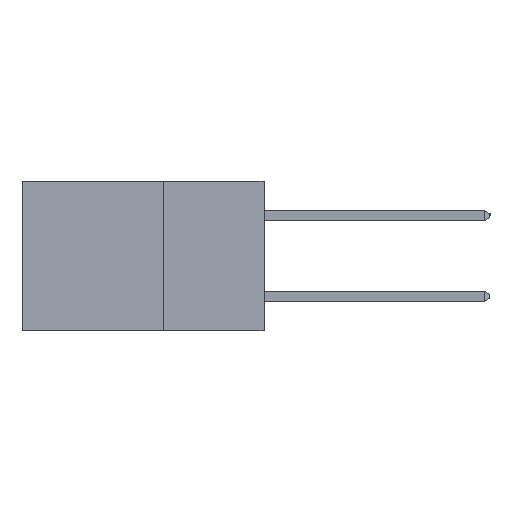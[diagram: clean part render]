
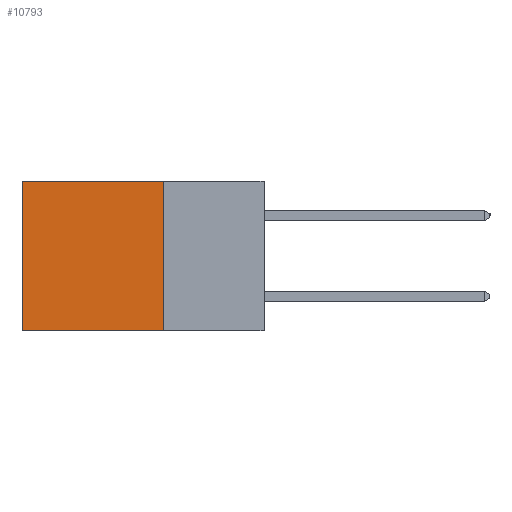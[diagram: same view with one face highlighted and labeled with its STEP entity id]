
A CAD part, left-side view. The second image highlights one B-rep face of the part: STEP entity #10793.
In plain terms, the highlighted planar face has unit normal (-1, 0, 0).
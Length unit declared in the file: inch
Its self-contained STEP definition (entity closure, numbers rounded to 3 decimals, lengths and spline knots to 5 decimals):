
#850 = VERTEX_POINT ( 'NONE', #3762 ) ;
#2221 = VECTOR ( 'NONE', #15880, 39.37008 ) ;
#2418 = CARTESIAN_POINT ( 'NONE',  ( 0.2615, 0.25, -0.37 ) ) ;
#2603 = ORIENTED_EDGE ( 'NONE', *, *, #13278, .T. ) ;
#2733 = ORIENTED_EDGE ( 'NONE', *, *, #13784, .T. ) ;
#2895 = VERTEX_POINT ( 'NONE', #5074 ) ;
#3762 = CARTESIAN_POINT ( 'NONE',  ( 0.2615, 0.25, 0. ) ) ;
#4779 = VERTEX_POINT ( 'NONE', #9271 ) ;
#4970 = CARTESIAN_POINT ( 'NONE',  ( 0.2615, 0.25, -0.37 ) ) ;
#5074 = CARTESIAN_POINT ( 'NONE',  ( 0.2615, 0.25, -0.37 ) ) ;
#6225 = LINE ( 'NONE', #11786, #14156 ) ;
#7426 = AXIS2_PLACEMENT_3D ( 'NONE', #8160, #14852, #13680 ) ;
#7540 = EDGE_CURVE ( 'NONE', #850, #2895, #10992, .T. ) ;
#8160 = CARTESIAN_POINT ( 'NONE',  ( 0.2615, 0.25, -0.37 ) ) ;
#9089 = LINE ( 'NONE', #10625, #2221 ) ;
#9271 = CARTESIAN_POINT ( 'NONE',  ( 0.2615, 0.6, -0.37 ) ) ;
#9443 = FACE_OUTER_BOUND ( 'NONE', #14579, .T. ) ;
#9508 = ORIENTED_EDGE ( 'NONE', *, *, #7540, .F. ) ;
#10090 = VECTOR ( 'NONE', #13066, 39.37008 ) ;
#10466 = VERTEX_POINT ( 'NONE', #11522 ) ;
#10625 = CARTESIAN_POINT ( 'NONE',  ( 0.2615, 0.6, -0.37 ) ) ;
#10630 = LINE ( 'NONE', #4970, #10090 ) ;
#10793 = ADVANCED_FACE ( 'NONE', ( #9443 ), #13589, .F. ) ;
#10992 = LINE ( 'NONE', #2418, #12883 ) ;
#11522 = CARTESIAN_POINT ( 'NONE',  ( 0.2615, 0.6, 0. ) ) ;
#11786 = CARTESIAN_POINT ( 'NONE',  ( 0.2615, 0.25, 0. ) ) ;
#12883 = VECTOR ( 'NONE', #13699, 39.37008 ) ;
#13066 = DIRECTION ( 'NONE',  ( 0., 1., 0. ) ) ;
#13278 = EDGE_CURVE ( 'NONE', #10466, #4779, #9089, .T. ) ;
#13589 = PLANE ( 'NONE',  #7426 ) ;
#13680 = DIRECTION ( 'NONE',  ( 0., 0., -1. ) ) ;
#13699 = DIRECTION ( 'NONE',  ( 0., 0., -1. ) ) ;
#13784 = EDGE_CURVE ( 'NONE', #850, #10466, #6225, .T. ) ;
#14156 = VECTOR ( 'NONE', #17408, 39.37008 ) ;
#14571 = EDGE_CURVE ( 'NONE', #2895, #4779, #10630, .T. ) ;
#14579 = EDGE_LOOP ( 'NONE', ( #2603, #16404, #9508, #2733 ) ) ;
#14852 = DIRECTION ( 'NONE',  ( 1., 0., 0. ) ) ;
#15880 = DIRECTION ( 'NONE',  ( 0., 0., -1. ) ) ;
#16404 = ORIENTED_EDGE ( 'NONE', *, *, #14571, .F. ) ;
#17408 = DIRECTION ( 'NONE',  ( 0., 1., 0. ) ) ;
